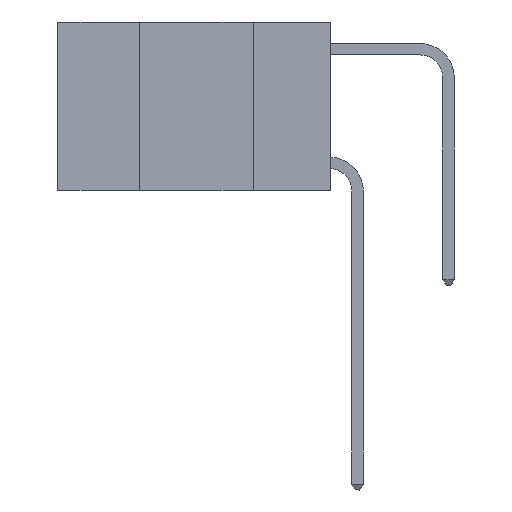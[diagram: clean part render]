
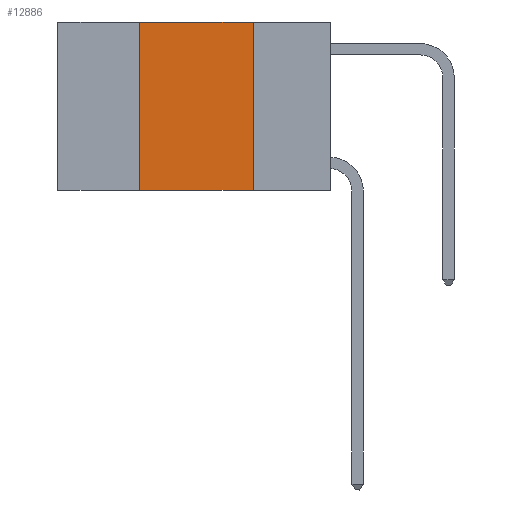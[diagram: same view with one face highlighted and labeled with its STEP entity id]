
A CAD part, left-side view. The second image highlights one B-rep face of the part: STEP entity #12886.
In plain terms, the highlighted planar face has unit normal (-1, 0, 0).
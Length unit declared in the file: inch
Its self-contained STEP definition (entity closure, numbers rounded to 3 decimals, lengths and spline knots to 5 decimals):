
#281 = CARTESIAN_POINT ( 'NONE',  ( 0., 0.6, 0. ) ) ;
#1306 = ORIENTED_EDGE ( 'NONE', *, *, #13991, .F. ) ;
#3018 = CARTESIAN_POINT ( 'NONE',  ( 0., 0.42, 0. ) ) ;
#3063 = AXIS2_PLACEMENT_3D ( 'NONE', #24885, #14872, #19029 ) ;
#3339 = VECTOR ( 'NONE', #14218, 39.37008 ) ;
#4359 = LINE ( 'NONE', #10460, #3339 ) ;
#5550 = VERTEX_POINT ( 'NONE', #13387 ) ;
#6940 = LINE ( 'NONE', #3018, #12612 ) ;
#8187 = DIRECTION ( 'NONE',  ( 0., -1., 0. ) ) ;
#8493 = CARTESIAN_POINT ( 'NONE',  ( 0., 0.17, -0.37 ) ) ;
#9353 = DIRECTION ( 'NONE',  ( 0., 0., -1. ) ) ;
#9748 = VECTOR ( 'NONE', #8187, 39.37008 ) ;
#10460 = CARTESIAN_POINT ( 'NONE',  ( 0., 0.6, -0.37 ) ) ;
#10816 = DIRECTION ( 'NONE',  ( 0., 0., 1. ) ) ;
#10862 = ORIENTED_EDGE ( 'NONE', *, *, #21514, .F. ) ;
#11100 = FACE_OUTER_BOUND ( 'NONE', #11547, .T. ) ;
#11547 = EDGE_LOOP ( 'NONE', ( #10862, #1306, #17176, #24105 ) ) ;
#12612 = VECTOR ( 'NONE', #10816, 39.37008 ) ;
#12886 = ADVANCED_FACE ( 'NONE', ( #11100 ), #21231, .F. ) ;
#13251 = EDGE_CURVE ( 'NONE', #5550, #21356, #6940, .T. ) ;
#13387 = CARTESIAN_POINT ( 'NONE',  ( 0., 0.42, -0.37 ) ) ;
#13490 = LINE ( 'NONE', #17387, #17001 ) ;
#13991 = EDGE_CURVE ( 'NONE', #21356, #19717, #24148, .T. ) ;
#14218 = DIRECTION ( 'NONE',  ( 0., -1., 0. ) ) ;
#14872 = DIRECTION ( 'NONE',  ( 1., 0., 0. ) ) ;
#16754 = CARTESIAN_POINT ( 'NONE',  ( 0., 0.42, 0. ) ) ;
#17001 = VECTOR ( 'NONE', #9353, 39.37008 ) ;
#17176 = ORIENTED_EDGE ( 'NONE', *, *, #13251, .F. ) ;
#17387 = CARTESIAN_POINT ( 'NONE',  ( 0., 0.17, 0. ) ) ;
#18735 = CARTESIAN_POINT ( 'NONE',  ( 0., 0.17, 0. ) ) ;
#19029 = DIRECTION ( 'NONE',  ( 0., 0., -1. ) ) ;
#19717 = VERTEX_POINT ( 'NONE', #18735 ) ;
#21231 = PLANE ( 'NONE',  #3063 ) ;
#21356 = VERTEX_POINT ( 'NONE', #16754 ) ;
#21514 = EDGE_CURVE ( 'NONE', #19717, #24406, #13490, .T. ) ;
#22114 = EDGE_CURVE ( 'NONE', #5550, #24406, #4359, .T. ) ;
#24105 = ORIENTED_EDGE ( 'NONE', *, *, #22114, .T. ) ;
#24148 = LINE ( 'NONE', #281, #9748 ) ;
#24406 = VERTEX_POINT ( 'NONE', #8493 ) ;
#24885 = CARTESIAN_POINT ( 'NONE',  ( 0., 0.6, 0. ) ) ;
